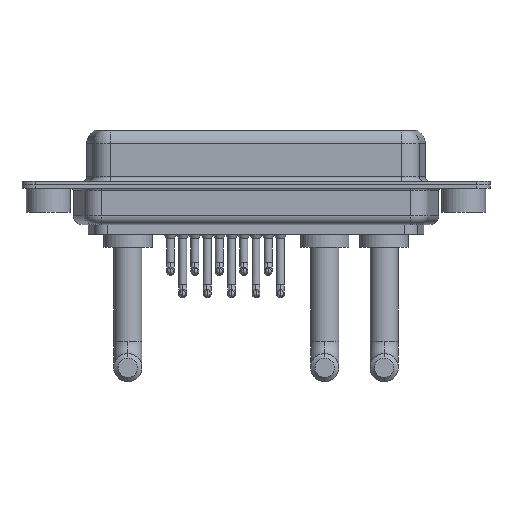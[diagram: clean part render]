
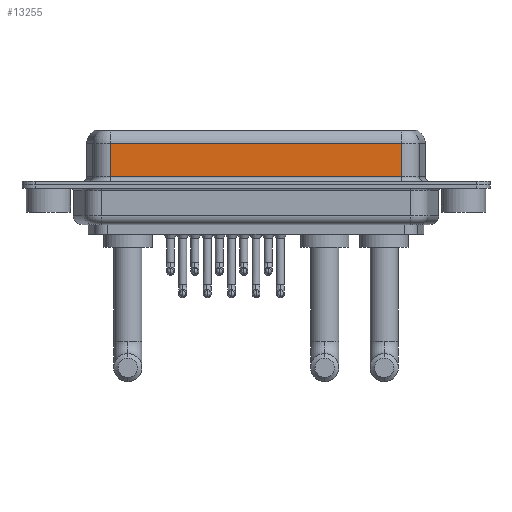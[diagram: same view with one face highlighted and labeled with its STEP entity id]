
A CAD part, front view. The second image highlights one B-rep face of the part: STEP entity #13255.
In plain terms, the highlighted planar face has unit normal (0, -1, 0).
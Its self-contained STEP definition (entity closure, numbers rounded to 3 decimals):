
#1671 = CARTESIAN_POINT ( 'NONE',  ( 40.037, -3.95, 0.9 ) ) ;
#2091 = CARTESIAN_POINT ( 'NONE',  ( 7.013, -3.95, 4.65 ) ) ;
#2299 = VERTEX_POINT ( 'NONE', #7521 ) ;
#2383 = LINE ( 'NONE', #8255, #18714 ) ;
#2482 = DIRECTION ( 'NONE',  ( 0., 0., -1. ) ) ;
#3329 = VERTEX_POINT ( 'NONE', #2091 ) ;
#3594 = DIRECTION ( 'NONE',  ( -1., 0., 0. ) ) ;
#4686 = EDGE_LOOP ( 'NONE', ( #11727, #9287, #6329, #9540 ) ) ;
#5142 = CARTESIAN_POINT ( 'NONE',  ( 40.037, -3.95, 4.65 ) ) ;
#5162 = VECTOR ( 'NONE', #18464, 1000. ) ;
#5197 = VERTEX_POINT ( 'NONE', #6778 ) ;
#5426 = AXIS2_PLACEMENT_3D ( 'NONE', #15013, #7486, #9325 ) ;
#5551 = VECTOR ( 'NONE', #3594, 1000. ) ;
#6164 = EDGE_CURVE ( 'NONE', #5197, #16072, #2383, .T. ) ;
#6329 = ORIENTED_EDGE ( 'NONE', *, *, #16073, .T. ) ;
#6677 = LINE ( 'NONE', #5142, #5551 ) ;
#6778 = CARTESIAN_POINT ( 'NONE',  ( 40.037, -3.95, 4.65 ) ) ;
#7248 = EDGE_CURVE ( 'NONE', #5197, #3329, #6677, .T. ) ;
#7486 = DIRECTION ( 'NONE',  ( 0., 1., 0. ) ) ;
#7521 = CARTESIAN_POINT ( 'NONE',  ( 7.013, -3.95, 0.9 ) ) ;
#8255 = CARTESIAN_POINT ( 'NONE',  ( 40.037, -3.95, 6.4 ) ) ;
#8536 = EDGE_CURVE ( 'NONE', #2299, #16072, #14850, .T. ) ;
#9287 = ORIENTED_EDGE ( 'NONE', *, *, #7248, .T. ) ;
#9325 = DIRECTION ( 'NONE',  ( 0., 0., 1. ) ) ;
#9540 = ORIENTED_EDGE ( 'NONE', *, *, #8536, .T. ) ;
#11247 = LINE ( 'NONE', #15860, #5162 ) ;
#11727 = ORIENTED_EDGE ( 'NONE', *, *, #6164, .F. ) ;
#13255 = ADVANCED_FACE ( 'NONE', ( #16655 ), #13363, .F. ) ;
#13363 = PLANE ( 'NONE',  #5426 ) ;
#13693 = DIRECTION ( 'NONE',  ( 1., 0., 0. ) ) ;
#14850 = LINE ( 'NONE', #1671, #16820 ) ;
#15013 = CARTESIAN_POINT ( 'NONE',  ( 40.037, -3.95, 6.4 ) ) ;
#15860 = CARTESIAN_POINT ( 'NONE',  ( 7.013, -3.95, 6.4 ) ) ;
#16072 = VERTEX_POINT ( 'NONE', #18374 ) ;
#16073 = EDGE_CURVE ( 'NONE', #3329, #2299, #11247, .T. ) ;
#16655 = FACE_OUTER_BOUND ( 'NONE', #4686, .T. ) ;
#16820 = VECTOR ( 'NONE', #13693, 1000. ) ;
#18374 = CARTESIAN_POINT ( 'NONE',  ( 40.037, -3.95, 0.9 ) ) ;
#18464 = DIRECTION ( 'NONE',  ( 0., 0., -1. ) ) ;
#18714 = VECTOR ( 'NONE', #2482, 1000. ) ;
